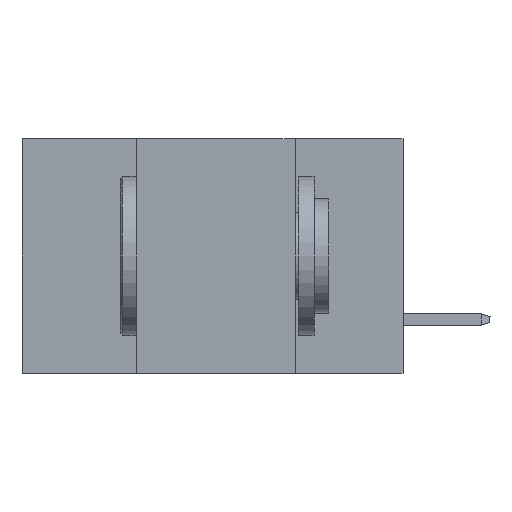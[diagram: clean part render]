
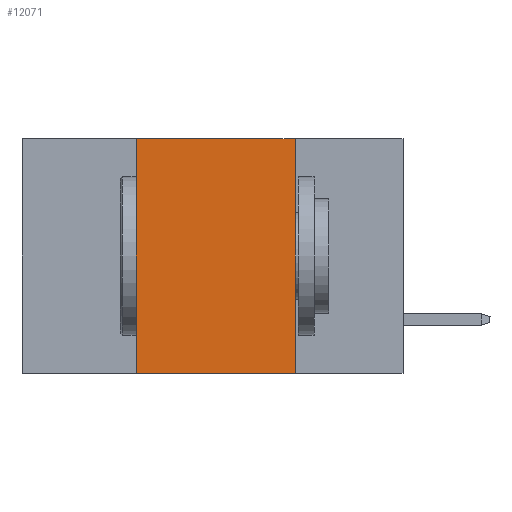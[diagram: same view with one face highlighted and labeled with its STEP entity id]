
A CAD part, left-side view. The second image highlights one B-rep face of the part: STEP entity #12071.
In plain terms, the highlighted planar face has unit normal (-1, 0, 0).
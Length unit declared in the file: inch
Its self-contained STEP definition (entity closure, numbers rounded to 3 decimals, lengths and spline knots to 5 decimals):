
#539 = LINE ( 'NONE', #6016, #16313 ) ;
#911 = EDGE_CURVE ( 'NONE', #30034, #10509, #539, .T. ) ;
#1062 = FACE_OUTER_BOUND ( 'NONE', #18599, .T. ) ;
#2151 = CARTESIAN_POINT ( 'NONE',  ( 0., 0.42, 0. ) ) ;
#3972 = VERTEX_POINT ( 'NONE', #19876 ) ;
#5762 = PLANE ( 'NONE',  #24017 ) ;
#6016 = CARTESIAN_POINT ( 'NONE',  ( 0., 0.17, 0. ) ) ;
#6057 = VECTOR ( 'NONE', #8076, 39.37008 ) ;
#6082 = DIRECTION ( 'NONE',  ( 1., 0., 0. ) ) ;
#6530 = ORIENTED_EDGE ( 'NONE', *, *, #31442, .F. ) ;
#6633 = ORIENTED_EDGE ( 'NONE', *, *, #911, .F. ) ;
#7250 = DIRECTION ( 'NONE',  ( 0., -1., 0. ) ) ;
#7370 = ORIENTED_EDGE ( 'NONE', *, *, #13245, .F. ) ;
#8076 = DIRECTION ( 'NONE',  ( 0., -1., 0. ) ) ;
#8307 = VECTOR ( 'NONE', #7250, 39.37008 ) ;
#9677 = LINE ( 'NONE', #9837, #8307 ) ;
#9721 = LINE ( 'NONE', #2151, #19954 ) ;
#9837 = CARTESIAN_POINT ( 'NONE',  ( 0., 0.6, 0. ) ) ;
#10382 = CARTESIAN_POINT ( 'NONE',  ( 0., 0.17, -0.37 ) ) ;
#10509 = VERTEX_POINT ( 'NONE', #10382 ) ;
#10929 = DIRECTION ( 'NONE',  ( 0., 0., -1. ) ) ;
#12071 = ADVANCED_FACE ( 'NONE', ( #1062 ), #5762, .F. ) ;
#13245 = EDGE_CURVE ( 'NONE', #3972, #28996, #9721, .T. ) ;
#14742 = EDGE_CURVE ( 'NONE', #3972, #10509, #25444, .T. ) ;
#14768 = CARTESIAN_POINT ( 'NONE',  ( 0., 0.42, 0. ) ) ;
#16313 = VECTOR ( 'NONE', #25338, 39.37008 ) ;
#17992 = CARTESIAN_POINT ( 'NONE',  ( 0., 0.6, 0. ) ) ;
#18599 = EDGE_LOOP ( 'NONE', ( #6633, #6530, #7370, #22072 ) ) ;
#19876 = CARTESIAN_POINT ( 'NONE',  ( 0., 0.42, -0.37 ) ) ;
#19954 = VECTOR ( 'NONE', #31477, 39.37008 ) ;
#22072 = ORIENTED_EDGE ( 'NONE', *, *, #14742, .T. ) ;
#24017 = AXIS2_PLACEMENT_3D ( 'NONE', #17992, #6082, #10929 ) ;
#25289 = CARTESIAN_POINT ( 'NONE',  ( 0., 0.6, -0.37 ) ) ;
#25338 = DIRECTION ( 'NONE',  ( 0., 0., -1. ) ) ;
#25444 = LINE ( 'NONE', #25289, #6057 ) ;
#28996 = VERTEX_POINT ( 'NONE', #14768 ) ;
#29142 = CARTESIAN_POINT ( 'NONE',  ( 0., 0.17, 0. ) ) ;
#30034 = VERTEX_POINT ( 'NONE', #29142 ) ;
#31442 = EDGE_CURVE ( 'NONE', #28996, #30034, #9677, .T. ) ;
#31477 = DIRECTION ( 'NONE',  ( 0., 0., 1. ) ) ;
